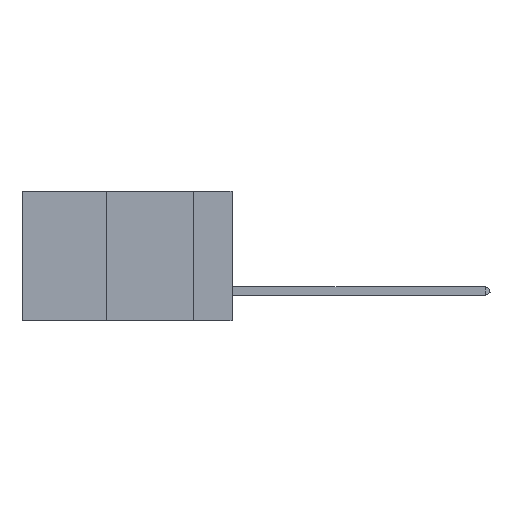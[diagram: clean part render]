
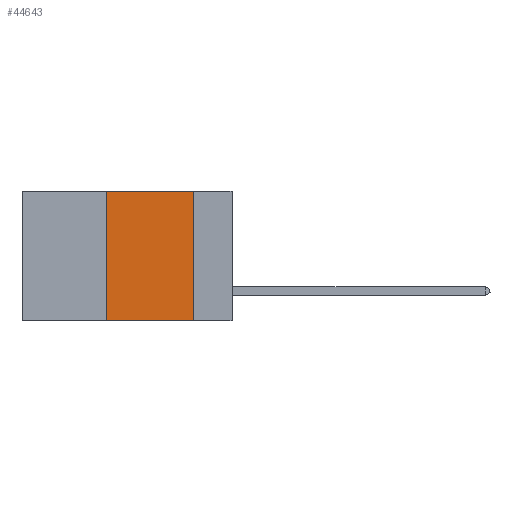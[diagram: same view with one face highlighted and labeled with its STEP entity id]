
A CAD part, left-side view. The second image highlights one B-rep face of the part: STEP entity #44643.
In plain terms, the highlighted planar face has unit normal (-1, 0, 0).
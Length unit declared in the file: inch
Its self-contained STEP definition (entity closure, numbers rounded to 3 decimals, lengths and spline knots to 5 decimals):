
#2448 = DIRECTION ( 'NONE',  ( 0., -1., 0. ) ) ;
#2659 = VERTEX_POINT ( 'NONE', #46105 ) ;
#5475 = EDGE_CURVE ( 'NONE', #33985, #2659, #31309, .T. ) ;
#5980 = DIRECTION ( 'NONE',  ( 0., 0., -1. ) ) ;
#9121 = ORIENTED_EDGE ( 'NONE', *, *, #44886, .T. ) ;
#9749 = VERTEX_POINT ( 'NONE', #30924 ) ;
#10211 = PLANE ( 'NONE',  #37364 ) ;
#11263 = LINE ( 'NONE', #20452, #32827 ) ;
#12106 = CARTESIAN_POINT ( 'NONE',  ( 0., 0.11, 0. ) ) ;
#13666 = DIRECTION ( 'NONE',  ( 0., 0., 1. ) ) ;
#14564 = LINE ( 'NONE', #21437, #30520 ) ;
#14615 = FACE_OUTER_BOUND ( 'NONE', #27129, .T. ) ;
#15241 = ORIENTED_EDGE ( 'NONE', *, *, #19354, .F. ) ;
#16357 = ORIENTED_EDGE ( 'NONE', *, *, #27529, .F. ) ;
#17068 = VECTOR ( 'NONE', #13666, 39.37008 ) ;
#19354 = EDGE_CURVE ( 'NONE', #2659, #40489, #11263, .T. ) ;
#20452 = CARTESIAN_POINT ( 'NONE',  ( 0., 0.6, 0. ) ) ;
#20671 = CARTESIAN_POINT ( 'NONE',  ( 0., 0.6, 0. ) ) ;
#21437 = CARTESIAN_POINT ( 'NONE',  ( 0., 0.6, -0.37 ) ) ;
#24437 = CARTESIAN_POINT ( 'NONE',  ( 0., 0.11, 0. ) ) ;
#26232 = DIRECTION ( 'NONE',  ( 0., 0., -1. ) ) ;
#26642 = CARTESIAN_POINT ( 'NONE',  ( 0., 0.36, -0.37 ) ) ;
#27129 = EDGE_LOOP ( 'NONE', ( #16357, #15241, #31706, #9121 ) ) ;
#27529 = EDGE_CURVE ( 'NONE', #40489, #9749, #45930, .T. ) ;
#30520 = VECTOR ( 'NONE', #36190, 39.37008 ) ;
#30924 = CARTESIAN_POINT ( 'NONE',  ( 0., 0.11, -0.37 ) ) ;
#31309 = LINE ( 'NONE', #31458, #17068 ) ;
#31458 = CARTESIAN_POINT ( 'NONE',  ( 0., 0.36, 0. ) ) ;
#31706 = ORIENTED_EDGE ( 'NONE', *, *, #5475, .F. ) ;
#32827 = VECTOR ( 'NONE', #2448, 39.37008 ) ;
#33985 = VERTEX_POINT ( 'NONE', #26642 ) ;
#36190 = DIRECTION ( 'NONE',  ( 0., -1., 0. ) ) ;
#37364 = AXIS2_PLACEMENT_3D ( 'NONE', #20671, #46039, #5980 ) ;
#40489 = VERTEX_POINT ( 'NONE', #24437 ) ;
#42516 = VECTOR ( 'NONE', #26232, 39.37008 ) ;
#44643 = ADVANCED_FACE ( 'NONE', ( #14615 ), #10211, .F. ) ;
#44886 = EDGE_CURVE ( 'NONE', #33985, #9749, #14564, .T. ) ;
#45930 = LINE ( 'NONE', #12106, #42516 ) ;
#46039 = DIRECTION ( 'NONE',  ( 1., 0., 0. ) ) ;
#46105 = CARTESIAN_POINT ( 'NONE',  ( 0., 0.36, 0. ) ) ;
